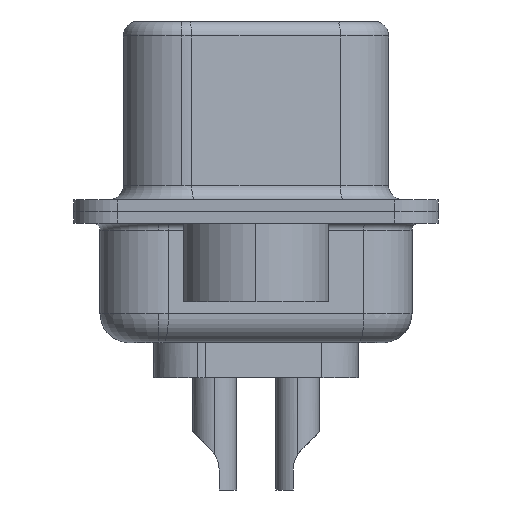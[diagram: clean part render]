
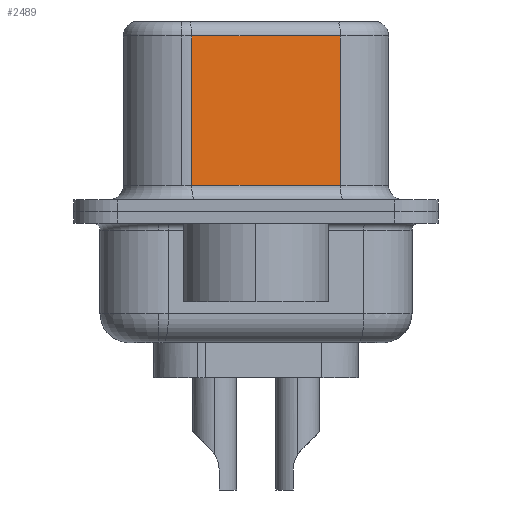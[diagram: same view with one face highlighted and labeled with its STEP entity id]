
A CAD part, left-side view. The second image highlights one B-rep face of the part: STEP entity #2489.
In plain terms, the highlighted planar face has unit normal (-0.985, -0.174, 0).
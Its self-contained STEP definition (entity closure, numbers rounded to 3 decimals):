
#391 = VECTOR ( 'NONE', #10092, 1000. ) ;
#796 = DIRECTION ( 'NONE',  ( 0., 0., -1. ) ) ;
#1275 = DIRECTION ( 'NONE',  ( -0.174, 0.985, 0. ) ) ;
#1470 = CARTESIAN_POINT ( 'NONE',  ( 3.655, 2.203, 6.52 ) ) ;
#1908 = ORIENTED_EDGE ( 'NONE', *, *, #6942, .F. ) ;
#2489 = ADVANCED_FACE ( 'NONE', ( #11934 ), #15740, .F. ) ;
#2571 = ORIENTED_EDGE ( 'NONE', *, *, #11725, .T. ) ;
#3212 = CARTESIAN_POINT ( 'NONE',  ( 4.555, -2.897, 6.52 ) ) ;
#3373 = CARTESIAN_POINT ( 'NONE',  ( 4.555, -2.897, 6.02 ) ) ;
#3444 = ORIENTED_EDGE ( 'NONE', *, *, #10133, .T. ) ;
#4345 = ORIENTED_EDGE ( 'NONE', *, *, #13004, .T. ) ;
#4792 = VERTEX_POINT ( 'NONE', #12955 ) ;
#4866 = CARTESIAN_POINT ( 'NONE',  ( 4.555, -2.897, 0.9 ) ) ;
#4927 = CARTESIAN_POINT ( 'NONE',  ( 3.655, 2.203, 0.9 ) ) ;
#6114 = CARTESIAN_POINT ( 'NONE',  ( 4.555, -2.897, 0.9 ) ) ;
#6942 = EDGE_CURVE ( 'NONE', #15668, #8612, #7331, .T. ) ;
#7172 = LINE ( 'NONE', #4866, #8937 ) ;
#7254 = VECTOR ( 'NONE', #17002, 1000. ) ;
#7282 = AXIS2_PLACEMENT_3D ( 'NONE', #10651, #9107, #1275 ) ;
#7331 = LINE ( 'NONE', #3212, #16838 ) ;
#8612 = VERTEX_POINT ( 'NONE', #6114 ) ;
#8937 = VECTOR ( 'NONE', #10120, 1000. ) ;
#9107 = DIRECTION ( 'NONE',  ( 0.985, 0.174, 0. ) ) ;
#10092 = DIRECTION ( 'NONE',  ( -0.174, 0.985, 0. ) ) ;
#10120 = DIRECTION ( 'NONE',  ( 0.174, -0.985, 0. ) ) ;
#10133 = EDGE_CURVE ( 'NONE', #15668, #4792, #12832, .T. ) ;
#10454 = CARTESIAN_POINT ( 'NONE',  ( 4.555, -2.897, 6.02 ) ) ;
#10651 = CARTESIAN_POINT ( 'NONE',  ( 4.555, -2.897, 6.52 ) ) ;
#10711 = EDGE_LOOP ( 'NONE', ( #1908, #3444, #2571, #4345 ) ) ;
#11725 = EDGE_CURVE ( 'NONE', #4792, #16084, #13263, .T. ) ;
#11934 = FACE_OUTER_BOUND ( 'NONE', #10711, .T. ) ;
#12832 = LINE ( 'NONE', #3373, #391 ) ;
#12955 = CARTESIAN_POINT ( 'NONE',  ( 3.655, 2.203, 6.02 ) ) ;
#13004 = EDGE_CURVE ( 'NONE', #16084, #8612, #7172, .T. ) ;
#13263 = LINE ( 'NONE', #1470, #7254 ) ;
#15668 = VERTEX_POINT ( 'NONE', #10454 ) ;
#15740 = PLANE ( 'NONE',  #7282 ) ;
#16084 = VERTEX_POINT ( 'NONE', #4927 ) ;
#16838 = VECTOR ( 'NONE', #796, 1000. ) ;
#17002 = DIRECTION ( 'NONE',  ( 0., 0., -1. ) ) ;
